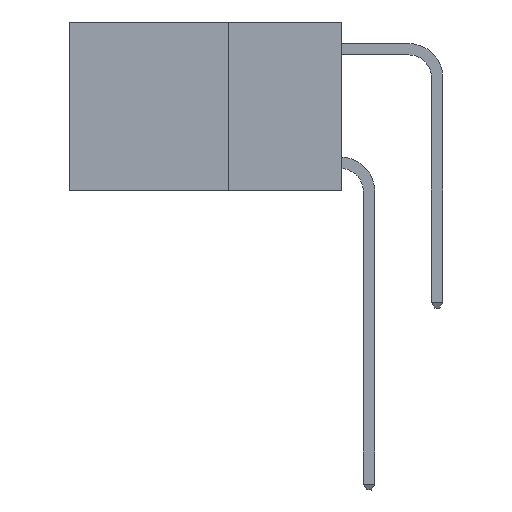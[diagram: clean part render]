
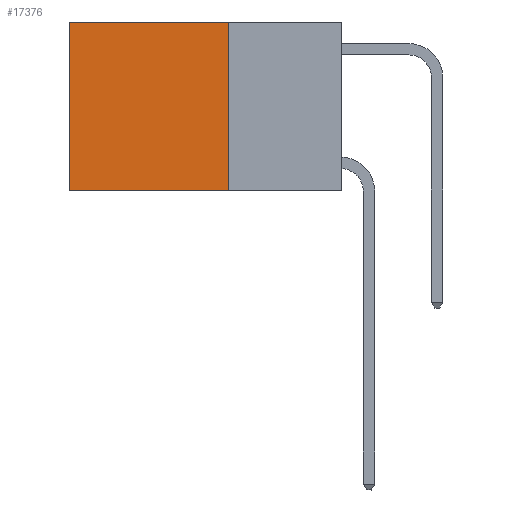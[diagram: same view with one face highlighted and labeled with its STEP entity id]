
A CAD part, left-side view. The second image highlights one B-rep face of the part: STEP entity #17376.
In plain terms, the highlighted planar face has unit normal (-1, 0, 0).
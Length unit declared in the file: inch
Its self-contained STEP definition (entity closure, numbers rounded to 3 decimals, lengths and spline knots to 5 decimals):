
#742 = VECTOR ( 'NONE', #11589, 39.37008 ) ;
#819 = DIRECTION ( 'NONE',  ( 0., 1., 0. ) ) ;
#1171 = LINE ( 'NONE', #10222, #742 ) ;
#1658 = EDGE_LOOP ( 'NONE', ( #8249, #5936, #3980, #6589 ) ) ;
#1833 = DIRECTION ( 'NONE',  ( 0., 1., 0. ) ) ;
#2041 = VECTOR ( 'NONE', #1833, 39.37008 ) ;
#2235 = CARTESIAN_POINT ( 'NONE',  ( 0.2625, 0.6, -0.37 ) ) ;
#2486 = LINE ( 'NONE', #16667, #2041 ) ;
#2687 = VECTOR ( 'NONE', #15651, 39.37008 ) ;
#3416 = VECTOR ( 'NONE', #819, 39.37008 ) ;
#3980 = ORIENTED_EDGE ( 'NONE', *, *, #9072, .F. ) ;
#4336 = VERTEX_POINT ( 'NONE', #9103 ) ;
#4386 = VERTEX_POINT ( 'NONE', #2235 ) ;
#4643 = PLANE ( 'NONE',  #13959 ) ;
#5936 = ORIENTED_EDGE ( 'NONE', *, *, #8519, .F. ) ;
#6022 = DIRECTION ( 'NONE',  ( 0., 0., -1. ) ) ;
#6589 = ORIENTED_EDGE ( 'NONE', *, *, #9023, .T. ) ;
#6859 = LINE ( 'NONE', #7799, #2687 ) ;
#7799 = CARTESIAN_POINT ( 'NONE',  ( 0.2625, 0.6, 0. ) ) ;
#8249 = ORIENTED_EDGE ( 'NONE', *, *, #15289, .T. ) ;
#8519 = EDGE_CURVE ( 'NONE', #10007, #4386, #14164, .T. ) ;
#8605 = CARTESIAN_POINT ( 'NONE',  ( 0.2625, 0.25, 0. ) ) ;
#9023 = EDGE_CURVE ( 'NONE', #9742, #4336, #2486, .T. ) ;
#9072 = EDGE_CURVE ( 'NONE', #9742, #10007, #1171, .T. ) ;
#9103 = CARTESIAN_POINT ( 'NONE',  ( 0.2625, 0.6, 0. ) ) ;
#9742 = VERTEX_POINT ( 'NONE', #11757 ) ;
#10007 = VERTEX_POINT ( 'NONE', #13679 ) ;
#10222 = CARTESIAN_POINT ( 'NONE',  ( 0.2625, 0.25, 0. ) ) ;
#11589 = DIRECTION ( 'NONE',  ( 0., 0., -1. ) ) ;
#11757 = CARTESIAN_POINT ( 'NONE',  ( 0.2625, 0.25, 0. ) ) ;
#11829 = FACE_OUTER_BOUND ( 'NONE', #1658, .T. ) ;
#13679 = CARTESIAN_POINT ( 'NONE',  ( 0.2625, 0.25, -0.37 ) ) ;
#13959 = AXIS2_PLACEMENT_3D ( 'NONE', #8605, #13994, #6022 ) ;
#13994 = DIRECTION ( 'NONE',  ( 1., 0., 0. ) ) ;
#14164 = LINE ( 'NONE', #14365, #3416 ) ;
#14365 = CARTESIAN_POINT ( 'NONE',  ( 0.2625, 0.25, -0.37 ) ) ;
#15289 = EDGE_CURVE ( 'NONE', #4336, #4386, #6859, .T. ) ;
#15651 = DIRECTION ( 'NONE',  ( 0., 0., -1. ) ) ;
#16667 = CARTESIAN_POINT ( 'NONE',  ( 0.2625, 0.25, 0. ) ) ;
#17376 = ADVANCED_FACE ( 'NONE', ( #11829 ), #4643, .F. ) ;
